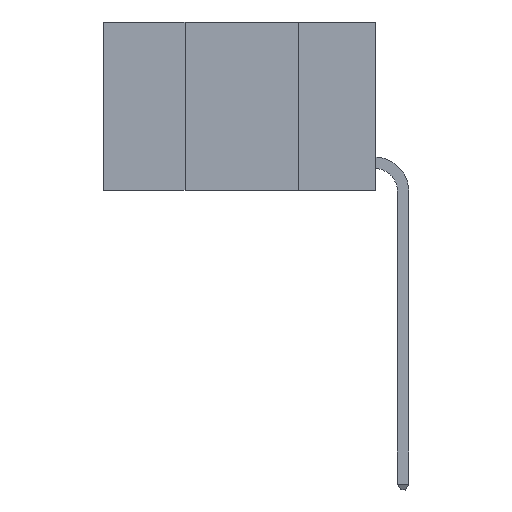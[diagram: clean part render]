
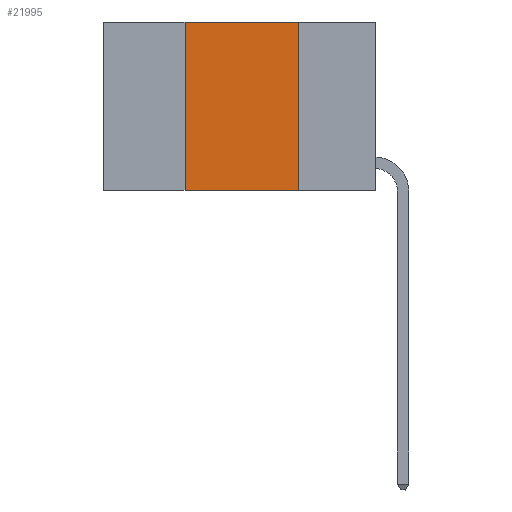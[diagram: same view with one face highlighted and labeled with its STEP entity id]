
A CAD part, left-side view. The second image highlights one B-rep face of the part: STEP entity #21995.
In plain terms, the highlighted planar face has unit normal (-1, 0, 0).
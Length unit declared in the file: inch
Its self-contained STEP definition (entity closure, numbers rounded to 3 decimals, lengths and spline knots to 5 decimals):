
#455 = CARTESIAN_POINT ( 'NONE',  ( 0., 0.6, -0.37 ) ) ;
#674 = DIRECTION ( 'NONE',  ( 0., -1., 0. ) ) ;
#1247 = ORIENTED_EDGE ( 'NONE', *, *, #17305, .T. ) ;
#1326 = AXIS2_PLACEMENT_3D ( 'NONE', #14101, #20462, #7823 ) ;
#3153 = DIRECTION ( 'NONE',  ( 0., 0., -1. ) ) ;
#3187 = ORIENTED_EDGE ( 'NONE', *, *, #6263, .F. ) ;
#3342 = ORIENTED_EDGE ( 'NONE', *, *, #10040, .F. ) ;
#3781 = VECTOR ( 'NONE', #11672, 39.37008 ) ;
#4841 = FACE_OUTER_BOUND ( 'NONE', #26913, .T. ) ;
#5414 = VERTEX_POINT ( 'NONE', #26838 ) ;
#6263 = EDGE_CURVE ( 'NONE', #6974, #5414, #25093, .T. ) ;
#6974 = VERTEX_POINT ( 'NONE', #11452 ) ;
#7726 = PLANE ( 'NONE',  #1326 ) ;
#7823 = DIRECTION ( 'NONE',  ( 0., 0., -1. ) ) ;
#9515 = CARTESIAN_POINT ( 'NONE',  ( 0., 0.17, -0.37 ) ) ;
#10040 = EDGE_CURVE ( 'NONE', #5414, #24815, #24702, .T. ) ;
#10355 = VERTEX_POINT ( 'NONE', #14710 ) ;
#11452 = CARTESIAN_POINT ( 'NONE',  ( 0., 0.42, 0. ) ) ;
#11578 = VECTOR ( 'NONE', #19557, 39.37008 ) ;
#11672 = DIRECTION ( 'NONE',  ( 0., 0., 1. ) ) ;
#12681 = VECTOR ( 'NONE', #674, 39.37008 ) ;
#13781 = CARTESIAN_POINT ( 'NONE',  ( 0., 0.42, 0. ) ) ;
#14101 = CARTESIAN_POINT ( 'NONE',  ( 0., 0.6, 0. ) ) ;
#14375 = LINE ( 'NONE', #13781, #3781 ) ;
#14710 = CARTESIAN_POINT ( 'NONE',  ( 0., 0.42, -0.37 ) ) ;
#17175 = LINE ( 'NONE', #455, #11578 ) ;
#17305 = EDGE_CURVE ( 'NONE', #10355, #24815, #17175, .T. ) ;
#19557 = DIRECTION ( 'NONE',  ( 0., -1., 0. ) ) ;
#19760 = CARTESIAN_POINT ( 'NONE',  ( 0., 0.6, 0. ) ) ;
#20462 = DIRECTION ( 'NONE',  ( 1., 0., 0. ) ) ;
#21983 = ORIENTED_EDGE ( 'NONE', *, *, #23011, .F. ) ;
#21995 = ADVANCED_FACE ( 'NONE', ( #4841 ), #7726, .F. ) ;
#23011 = EDGE_CURVE ( 'NONE', #10355, #6974, #14375, .T. ) ;
#24048 = VECTOR ( 'NONE', #3153, 39.37008 ) ;
#24702 = LINE ( 'NONE', #26185, #24048 ) ;
#24815 = VERTEX_POINT ( 'NONE', #9515 ) ;
#25093 = LINE ( 'NONE', #19760, #12681 ) ;
#26185 = CARTESIAN_POINT ( 'NONE',  ( 0., 0.17, 0. ) ) ;
#26838 = CARTESIAN_POINT ( 'NONE',  ( 0., 0.17, 0. ) ) ;
#26913 = EDGE_LOOP ( 'NONE', ( #3342, #3187, #21983, #1247 ) ) ;
